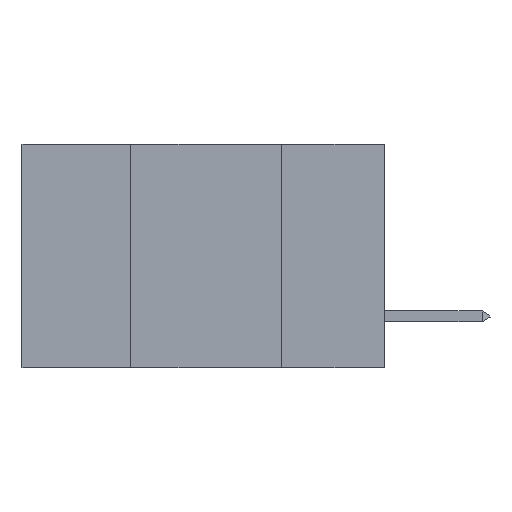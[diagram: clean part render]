
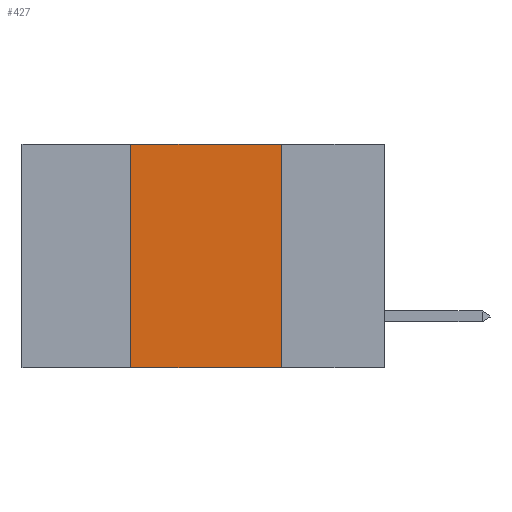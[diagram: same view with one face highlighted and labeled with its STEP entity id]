
A CAD part, left-side view. The second image highlights one B-rep face of the part: STEP entity #427.
In plain terms, the highlighted planar face has unit normal (-1, 0, 0).
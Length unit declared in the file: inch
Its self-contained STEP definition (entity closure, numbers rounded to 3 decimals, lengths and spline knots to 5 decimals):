
#427 = ADVANCED_FACE ( 'NONE', ( #3069 ), #1817, .F. ) ;
#473 = CARTESIAN_POINT ( 'NONE',  ( 0., 0.6, -0.37 ) ) ;
#891 = VECTOR ( 'NONE', #1707, 39.37008 ) ;
#1166 = CARTESIAN_POINT ( 'NONE',  ( 0., 0.17, -0.37 ) ) ;
#1707 = DIRECTION ( 'NONE',  ( 0., 0., 1. ) ) ;
#1817 = PLANE ( 'NONE',  #3053 ) ;
#2370 = LINE ( 'NONE', #6855, #891 ) ;
#2637 = EDGE_LOOP ( 'NONE', ( #9673, #4746, #10855, #3852 ) ) ;
#3053 = AXIS2_PLACEMENT_3D ( 'NONE', #9027, #3961, #5178 ) ;
#3069 = FACE_OUTER_BOUND ( 'NONE', #2637, .T. ) ;
#3197 = EDGE_CURVE ( 'NONE', #5393, #6678, #2370, .T. ) ;
#3606 = VERTEX_POINT ( 'NONE', #1166 ) ;
#3852 = ORIENTED_EDGE ( 'NONE', *, *, #9227, .T. ) ;
#3961 = DIRECTION ( 'NONE',  ( 1., 0., 0. ) ) ;
#4187 = CARTESIAN_POINT ( 'NONE',  ( 0., 0.42, -0.37 ) ) ;
#4679 = LINE ( 'NONE', #473, #5799 ) ;
#4697 = VECTOR ( 'NONE', #11407, 39.37008 ) ;
#4746 = ORIENTED_EDGE ( 'NONE', *, *, #6294, .F. ) ;
#5178 = DIRECTION ( 'NONE',  ( 0., 0., -1. ) ) ;
#5386 = CARTESIAN_POINT ( 'NONE',  ( 0., 0.17, 0. ) ) ;
#5393 = VERTEX_POINT ( 'NONE', #4187 ) ;
#5799 = VECTOR ( 'NONE', #7746, 39.37008 ) ;
#6294 = EDGE_CURVE ( 'NONE', #6678, #10749, #9490, .T. ) ;
#6678 = VERTEX_POINT ( 'NONE', #7416 ) ;
#6696 = LINE ( 'NONE', #8727, #9070 ) ;
#6822 = DIRECTION ( 'NONE',  ( 0., 0., -1. ) ) ;
#6855 = CARTESIAN_POINT ( 'NONE',  ( 0., 0.42, 0. ) ) ;
#7272 = CARTESIAN_POINT ( 'NONE',  ( 0., 0.6, 0. ) ) ;
#7416 = CARTESIAN_POINT ( 'NONE',  ( 0., 0.42, 0. ) ) ;
#7746 = DIRECTION ( 'NONE',  ( 0., -1., 0. ) ) ;
#8727 = CARTESIAN_POINT ( 'NONE',  ( 0., 0.17, 0. ) ) ;
#9027 = CARTESIAN_POINT ( 'NONE',  ( 0., 0.6, 0. ) ) ;
#9070 = VECTOR ( 'NONE', #6822, 39.37008 ) ;
#9227 = EDGE_CURVE ( 'NONE', #5393, #3606, #4679, .T. ) ;
#9490 = LINE ( 'NONE', #7272, #4697 ) ;
#9673 = ORIENTED_EDGE ( 'NONE', *, *, #12164, .F. ) ;
#10749 = VERTEX_POINT ( 'NONE', #5386 ) ;
#10855 = ORIENTED_EDGE ( 'NONE', *, *, #3197, .F. ) ;
#11407 = DIRECTION ( 'NONE',  ( 0., -1., 0. ) ) ;
#12164 = EDGE_CURVE ( 'NONE', #10749, #3606, #6696, .T. ) ;
